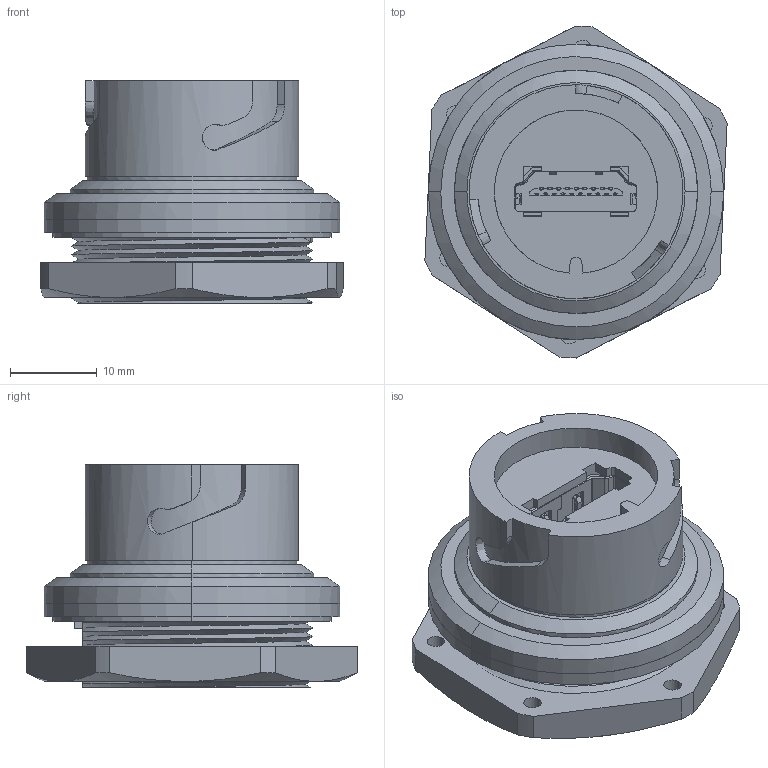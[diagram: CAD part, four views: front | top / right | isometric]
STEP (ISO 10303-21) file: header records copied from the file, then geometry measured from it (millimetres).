
FILE_DESCRIPTION (( 'STEP AP214' ), '1' );
FILE_NAME ('694-W19-260-015.STEP', '2021-07-13T13:22:23', ( '' ), ( '' ), 'SwSTEP 2.0', 'SolidWorks 2020', '' );
FILE_SCHEMA (( 'AUTOMOTIVE_DESIGN' ));
Length unit declared in the file: millimetre
Products named in the file (11): 694-W19-260-015; HOUSING 694-W19-X60-015; HDMI ASSY 694-W19-X60-015; RING 694-W19-X60-015; HDMI HOUSING1 694-W19-X60-015; HDMI CONTACT2 694-W19-X60-015; HDMI CONTACT1 694-W19-X60-015; LOCK NUT 694-W19-X60-015; HDMI SHELL 694-W19-X60-015; O-RING 694-W19-X60-015; HDMI HOUSING2 694-W19-X60-015
Assembly tree (27 placements, depth 3):
  694-W19-260-015
    HDMI ASSY 694-W19-X60-015
      HDMI HOUSING1 694-W19-X60-015
      HDMI HOUSING2 694-W19-X60-015
      HDMI CONTACT1 694-W19-X60-015  x9
      HDMI CONTACT2 694-W19-X60-015  x10
      HDMI SHELL 694-W19-X60-015
    HOUSING 694-W19-X60-015
    O-RING 694-W19-X60-015
    RING 694-W19-X60-015
    LOCK NUT 694-W19-X60-015
Bounding box: 34.78 x 38.2 x 25.6 mm (x, y, z)
Volume: 9559 mm3; surface area: 12979.8 mm2
Topology: 26 solids, 26 shells, 2027 faces, 5889 edges, 3886 vertices
Faces by surface type: plane 1388, cylinder 574, bspline 45, cone 20
Entity records: 50331 total; most frequent: CARTESIAN_POINT 20185, ORIENTED_EDGE 6678, DIRECTION 5380, EDGE_CURVE 3339, LINE 2660, VECTOR 2660, VERTEX_POINT 2186, AXIS2_PLACEMENT_3D 1360
